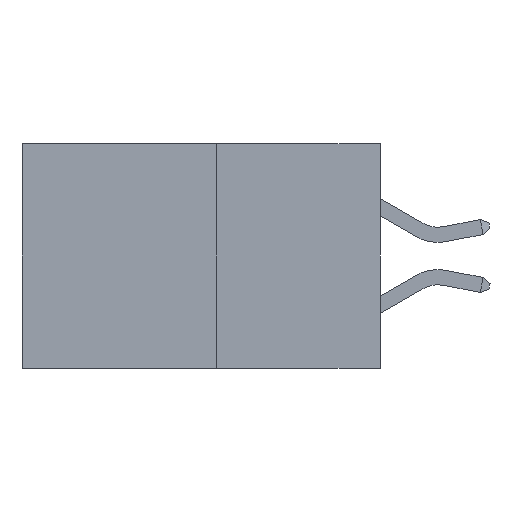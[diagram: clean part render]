
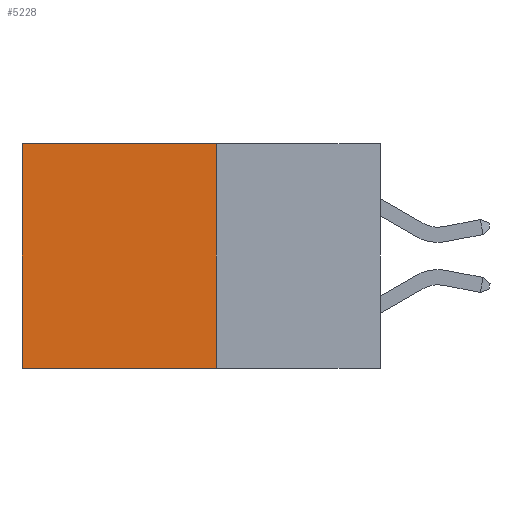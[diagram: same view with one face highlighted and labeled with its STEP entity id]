
A CAD part, left-side view. The second image highlights one B-rep face of the part: STEP entity #5228.
In plain terms, the highlighted planar face has unit normal (-1, 0, 0).
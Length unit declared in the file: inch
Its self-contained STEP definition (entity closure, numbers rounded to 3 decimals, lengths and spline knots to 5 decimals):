
#151 = VECTOR ( 'NONE', #1406, 39.37008 ) ;
#265 = CARTESIAN_POINT ( 'NONE',  ( 0.277, 0.59, -0.37 ) ) ;
#295 = VECTOR ( 'NONE', #3929, 39.37008 ) ;
#772 = EDGE_CURVE ( 'NONE', #10642, #1024, #10563, .T. ) ;
#1024 = VERTEX_POINT ( 'NONE', #1648 ) ;
#1405 = CARTESIAN_POINT ( 'NONE',  ( 0.277, 0.27, -0.37 ) ) ;
#1406 = DIRECTION ( 'NONE',  ( 0., 1., 0. ) ) ;
#1648 = CARTESIAN_POINT ( 'NONE',  ( 0.277, 0.59, 0. ) ) ;
#1900 = LINE ( 'NONE', #2705, #4643 ) ;
#2174 = ORIENTED_EDGE ( 'NONE', *, *, #8951, .T. ) ;
#2324 = ORIENTED_EDGE ( 'NONE', *, *, #7526, .F. ) ;
#2483 = DIRECTION ( 'NONE',  ( 0., 0., -1. ) ) ;
#2576 = DIRECTION ( 'NONE',  ( 0., 1., 0. ) ) ;
#2705 = CARTESIAN_POINT ( 'NONE',  ( 0.277, 0.27, -0.37 ) ) ;
#3169 = VERTEX_POINT ( 'NONE', #11648 ) ;
#3459 = DIRECTION ( 'NONE',  ( 0., 0., -1. ) ) ;
#3929 = DIRECTION ( 'NONE',  ( 0., 0., -1. ) ) ;
#4283 = PLANE ( 'NONE',  #8437 ) ;
#4357 = VERTEX_POINT ( 'NONE', #4543 ) ;
#4543 = CARTESIAN_POINT ( 'NONE',  ( 0.277, 0.27, -0.37 ) ) ;
#4638 = EDGE_CURVE ( 'NONE', #4357, #3169, #1900, .T. ) ;
#4643 = VECTOR ( 'NONE', #2576, 39.37008 ) ;
#5152 = EDGE_LOOP ( 'NONE', ( #2174, #9970, #2324, #7695 ) ) ;
#5228 = ADVANCED_FACE ( 'NONE', ( #6346 ), #4283, .F. ) ;
#6346 = FACE_OUTER_BOUND ( 'NONE', #5152, .T. ) ;
#7526 = EDGE_CURVE ( 'NONE', #10642, #4357, #11277, .T. ) ;
#7695 = ORIENTED_EDGE ( 'NONE', *, *, #772, .T. ) ;
#8012 = CARTESIAN_POINT ( 'NONE',  ( 0.277, 0.27, 0. ) ) ;
#8408 = LINE ( 'NONE', #265, #10659 ) ;
#8437 = AXIS2_PLACEMENT_3D ( 'NONE', #1405, #8496, #2483 ) ;
#8496 = DIRECTION ( 'NONE',  ( 1., 0., 0. ) ) ;
#8879 = CARTESIAN_POINT ( 'NONE',  ( 0.277, 0.27, -0.37 ) ) ;
#8951 = EDGE_CURVE ( 'NONE', #1024, #3169, #8408, .T. ) ;
#9970 = ORIENTED_EDGE ( 'NONE', *, *, #4638, .F. ) ;
#10146 = CARTESIAN_POINT ( 'NONE',  ( 0.277, 0.27, 0. ) ) ;
#10563 = LINE ( 'NONE', #10146, #151 ) ;
#10642 = VERTEX_POINT ( 'NONE', #8012 ) ;
#10659 = VECTOR ( 'NONE', #3459, 39.37008 ) ;
#11277 = LINE ( 'NONE', #8879, #295 ) ;
#11648 = CARTESIAN_POINT ( 'NONE',  ( 0.277, 0.59, -0.37 ) ) ;
